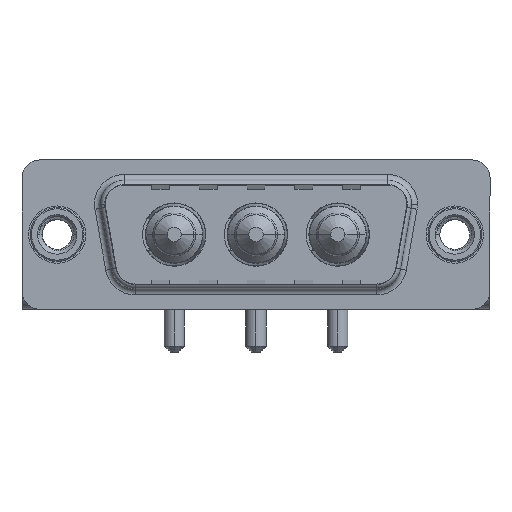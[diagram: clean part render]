
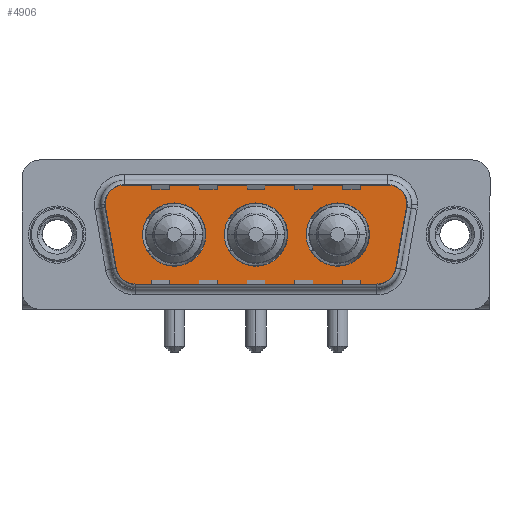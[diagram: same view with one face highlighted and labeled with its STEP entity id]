
A CAD part, top view. The second image highlights one B-rep face of the part: STEP entity #4906.
In plain terms, the highlighted planar face has unit normal (0, 0, 1).
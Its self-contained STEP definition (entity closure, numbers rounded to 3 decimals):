
#16 = DIRECTION ( 'NONE',  ( -1., 0., 0. ) ) ;
#33 = PLANE ( 'NONE',  #1179 ) ;
#123 = DIRECTION ( 'NONE',  ( 0., 0., 1. ) ) ;
#178 = CARTESIAN_POINT ( 'NONE',  ( 6.434, -4.9, 0. ) ) ;
#277 = CIRCLE ( 'NONE', #11703, 2.65 ) ;
#306 = EDGE_CURVE ( 'NONE', #2832, #10535, #11459, .T. ) ;
#308 = EDGE_LOOP ( 'NONE', ( #3486, #2966 ) ) ;
#318 = EDGE_CURVE ( 'NONE', #6557, #2832, #5088, .T. ) ;
#362 = DIRECTION ( 'NONE',  ( -1., 0., 0. ) ) ;
#555 = CARTESIAN_POINT ( 'NONE',  ( 20.85, 0., 0. ) ) ;
#577 = VERTEX_POINT ( 'NONE', #15387 ) ;
#631 = CARTESIAN_POINT ( 'NONE',  ( 5.411, 4.9, 0. ) ) ;
#693 = ORIENTED_EDGE ( 'NONE', *, *, #10812, .F. ) ;
#882 = VERTEX_POINT ( 'NONE', #12918 ) ;
#958 = ORIENTED_EDGE ( 'NONE', *, *, #3874, .T. ) ;
#1175 = ORIENTED_EDGE ( 'NONE', *, *, #6913, .T. ) ;
#1179 = AXIS2_PLACEMENT_3D ( 'NONE', #11768, #9429, #8314 ) ;
#1227 = CARTESIAN_POINT ( 'NONE',  ( 9.8, 0., 0. ) ) ;
#1239 = EDGE_CURVE ( 'NONE', #577, #13368, #1849, .T. ) ;
#1343 = VECTOR ( 'NONE', #4263, 1000. ) ;
#1418 = AXIS2_PLACEMENT_3D ( 'NONE', #13513, #1530, #4067 ) ;
#1456 = DIRECTION ( 'NONE',  ( 1., 0., 0. ) ) ;
#1499 = VERTEX_POINT ( 'NONE', #13284 ) ;
#1530 = DIRECTION ( 'NONE',  ( 0., 0., 1. ) ) ;
#1849 = LINE ( 'NONE', #10267, #1343 ) ;
#1868 = CARTESIAN_POINT ( 'NONE',  ( 16.65, 0., 0. ) ) ;
#1875 = EDGE_CURVE ( 'NONE', #1499, #2037, #9736, .T. ) ;
#2017 = CARTESIAN_POINT ( 'NONE',  ( 27.889, 2.9, 0. ) ) ;
#2037 = VERTEX_POINT ( 'NONE', #4040 ) ;
#2110 = DIRECTION ( 'NONE',  ( 1., 0., 0. ) ) ;
#2243 = DIRECTION ( 'NONE',  ( 0., 0., 1. ) ) ;
#2262 = EDGE_CURVE ( 'NONE', #4130, #882, #277, .T. ) ;
#2265 = EDGE_CURVE ( 'NONE', #13368, #1499, #2493, .T. ) ;
#2266 = FACE_BOUND ( 'NONE', #13736, .T. ) ;
#2382 = CIRCLE ( 'NONE', #14342, 2. ) ;
#2460 = VERTEX_POINT ( 'NONE', #3016 ) ;
#2493 = CIRCLE ( 'NONE', #14206, 2. ) ;
#2589 = ORIENTED_EDGE ( 'NONE', *, *, #1239, .T. ) ;
#2832 = VERTEX_POINT ( 'NONE', #9776 ) ;
#2833 = CARTESIAN_POINT ( 'NONE',  ( 27.889, 2.9, 0. ) ) ;
#2956 = VERTEX_POINT ( 'NONE', #6421 ) ;
#2966 = ORIENTED_EDGE ( 'NONE', *, *, #6146, .F. ) ;
#3016 = CARTESIAN_POINT ( 'NONE',  ( 27.889, 4.9, 0. ) ) ;
#3232 = VECTOR ( 'NONE', #11190, 1000. ) ;
#3486 = ORIENTED_EDGE ( 'NONE', *, *, #13409, .F. ) ;
#3497 = ORIENTED_EDGE ( 'NONE', *, *, #4980, .T. ) ;
#3520 = ORIENTED_EDGE ( 'NONE', *, *, #2262, .F. ) ;
#3670 = CARTESIAN_POINT ( 'NONE',  ( 29.889, 2.9, 0. ) ) ;
#3732 = CARTESIAN_POINT ( 'NONE',  ( 9.8, 0., 0. ) ) ;
#3874 = EDGE_CURVE ( 'NONE', #10535, #2460, #2382, .T. ) ;
#4016 = CARTESIAN_POINT ( 'NONE',  ( 12.45, 0., 0. ) ) ;
#4040 = CARTESIAN_POINT ( 'NONE',  ( 26.866, -4.9, 0. ) ) ;
#4067 = DIRECTION ( 'NONE',  ( 1., 0., 0. ) ) ;
#4130 = VERTEX_POINT ( 'NONE', #7362 ) ;
#4263 = DIRECTION ( 'NONE',  ( 0.174, -0.985, 0. ) ) ;
#4637 = AXIS2_PLACEMENT_3D ( 'NONE', #1227, #10951, #1456 ) ;
#4663 = DIRECTION ( 'NONE',  ( 0., 0., 1. ) ) ;
#4906 = ADVANCED_FACE ( 'NONE', ( #10449, #2266, #8177, #8095 ), #33, .T. ) ;
#4966 = AXIS2_PLACEMENT_3D ( 'NONE', #2833, #8903, #362 ) ;
#4980 = EDGE_CURVE ( 'NONE', #2037, #6557, #6131, .T. ) ;
#5088 = LINE ( 'NONE', #8590, #3232 ) ;
#5361 = VERTEX_POINT ( 'NONE', #631 ) ;
#5397 = CARTESIAN_POINT ( 'NONE',  ( 28.836, -3.247, 0. ) ) ;
#5449 = DIRECTION ( 'NONE',  ( 1., 0., 0. ) ) ;
#5856 = CARTESIAN_POINT ( 'NONE',  ( 5.411, 4.9, 0. ) ) ;
#5874 = CIRCLE ( 'NONE', #1418, 2.65 ) ;
#6131 = CIRCLE ( 'NONE', #14111, 2. ) ;
#6146 = EDGE_CURVE ( 'NONE', #2956, #7357, #10863, .T. ) ;
#6311 = EDGE_CURVE ( 'NONE', #14594, #9166, #5874, .T. ) ;
#6421 = CARTESIAN_POINT ( 'NONE',  ( 7.15, 0., 0. ) ) ;
#6469 = EDGE_LOOP ( 'NONE', ( #3497, #14538, #8035, #958, #12349, #1175, #2589, #9336, #13315 ) ) ;
#6557 = VERTEX_POINT ( 'NONE', #5397 ) ;
#6587 = CIRCLE ( 'NONE', #15316, 2.65 ) ;
#6913 = EDGE_CURVE ( 'NONE', #5361, #577, #10352, .T. ) ;
#7357 = VERTEX_POINT ( 'NONE', #4016 ) ;
#7362 = CARTESIAN_POINT ( 'NONE',  ( 19.3, 0., 0. ) ) ;
#7737 = CARTESIAN_POINT ( 'NONE',  ( 26.15, 0., 0. ) ) ;
#8035 = ORIENTED_EDGE ( 'NONE', *, *, #306, .T. ) ;
#8095 = FACE_OUTER_BOUND ( 'NONE', #6469, .T. ) ;
#8177 = FACE_BOUND ( 'NONE', #308, .T. ) ;
#8199 = DIRECTION ( 'NONE',  ( 1., 0., 0. ) ) ;
#8230 = CARTESIAN_POINT ( 'NONE',  ( 6.434, -2.9, 0. ) ) ;
#8314 = DIRECTION ( 'NONE',  ( 1., 0., 0. ) ) ;
#8431 = LINE ( 'NONE', #5856, #13639 ) ;
#8543 = EDGE_CURVE ( 'NONE', #2460, #5361, #8431, .T. ) ;
#8590 = CARTESIAN_POINT ( 'NONE',  ( 29.859, 2.553, 0. ) ) ;
#8716 = DIRECTION ( 'NONE',  ( 1., 0., 0. ) ) ;
#8863 = CIRCLE ( 'NONE', #11377, 2.65 ) ;
#8903 = DIRECTION ( 'NONE',  ( 0., 0., 1. ) ) ;
#9166 = VERTEX_POINT ( 'NONE', #555 ) ;
#9177 = AXIS2_PLACEMENT_3D ( 'NONE', #11794, #123, #8199 ) ;
#9179 = DIRECTION ( 'NONE',  ( 0., 0., 1. ) ) ;
#9336 = ORIENTED_EDGE ( 'NONE', *, *, #2265, .T. ) ;
#9412 = DIRECTION ( 'NONE',  ( 1., 0., 0. ) ) ;
#9429 = DIRECTION ( 'NONE',  ( 0., 0., 1. ) ) ;
#9504 = CARTESIAN_POINT ( 'NONE',  ( 26.866, -2.9, 0. ) ) ;
#9736 = LINE ( 'NONE', #178, #13416 ) ;
#9776 = CARTESIAN_POINT ( 'NONE',  ( 29.859, 2.553, 0. ) ) ;
#9987 = EDGE_LOOP ( 'NONE', ( #3520, #693 ) ) ;
#10070 = EDGE_CURVE ( 'NONE', #9166, #14594, #10682, .T. ) ;
#10267 = CARTESIAN_POINT ( 'NONE',  ( 3.441, 2.553, 0. ) ) ;
#10352 = CIRCLE ( 'NONE', #13861, 2. ) ;
#10449 = FACE_BOUND ( 'NONE', #9987, .T. ) ;
#10535 = VERTEX_POINT ( 'NONE', #3670 ) ;
#10663 = DIRECTION ( 'NONE',  ( 1., 0., 0. ) ) ;
#10682 = CIRCLE ( 'NONE', #9177, 2.65 ) ;
#10812 = EDGE_CURVE ( 'NONE', #882, #4130, #6587, .T. ) ;
#10863 = CIRCLE ( 'NONE', #4637, 2.65 ) ;
#10951 = DIRECTION ( 'NONE',  ( 0., 0., 1. ) ) ;
#10984 = DIRECTION ( 'NONE',  ( 1., 0., 0. ) ) ;
#11123 = ORIENTED_EDGE ( 'NONE', *, *, #10070, .F. ) ;
#11190 = DIRECTION ( 'NONE',  ( 0.174, 0.985, 0. ) ) ;
#11377 = AXIS2_PLACEMENT_3D ( 'NONE', #3732, #13165, #10984 ) ;
#11459 = CIRCLE ( 'NONE', #4966, 2. ) ;
#11703 = AXIS2_PLACEMENT_3D ( 'NONE', #15348, #4663, #9412 ) ;
#11768 = CARTESIAN_POINT ( 'NONE',  ( 26.866, -2.9, 0. ) ) ;
#11794 = CARTESIAN_POINT ( 'NONE',  ( 23.5, 0., 0. ) ) ;
#11882 = DIRECTION ( 'NONE',  ( -1., 0., 0. ) ) ;
#12349 = ORIENTED_EDGE ( 'NONE', *, *, #8543, .T. ) ;
#12639 = CARTESIAN_POINT ( 'NONE',  ( 5.411, 2.9, 0. ) ) ;
#12709 = DIRECTION ( 'NONE',  ( 0., 0., 1. ) ) ;
#12918 = CARTESIAN_POINT ( 'NONE',  ( 14., 0., 0. ) ) ;
#13010 = DIRECTION ( 'NONE',  ( 0., 0., 1. ) ) ;
#13165 = DIRECTION ( 'NONE',  ( 0., 0., 1. ) ) ;
#13284 = CARTESIAN_POINT ( 'NONE',  ( 6.434, -4.9, 0. ) ) ;
#13315 = ORIENTED_EDGE ( 'NONE', *, *, #1875, .T. ) ;
#13368 = VERTEX_POINT ( 'NONE', #15042 ) ;
#13409 = EDGE_CURVE ( 'NONE', #7357, #2956, #8863, .T. ) ;
#13416 = VECTOR ( 'NONE', #8716, 1000. ) ;
#13429 = ORIENTED_EDGE ( 'NONE', *, *, #6311, .F. ) ;
#13513 = CARTESIAN_POINT ( 'NONE',  ( 23.5, 0., 0. ) ) ;
#13631 = DIRECTION ( 'NONE',  ( 0., 0., 1. ) ) ;
#13639 = VECTOR ( 'NONE', #11882, 1000. ) ;
#13736 = EDGE_LOOP ( 'NONE', ( #13429, #11123 ) ) ;
#13784 = DIRECTION ( 'NONE',  ( -1., 0., 0. ) ) ;
#13861 = AXIS2_PLACEMENT_3D ( 'NONE', #12639, #2243, #10663 ) ;
#14111 = AXIS2_PLACEMENT_3D ( 'NONE', #9504, #13010, #2110 ) ;
#14206 = AXIS2_PLACEMENT_3D ( 'NONE', #8230, #9179, #16 ) ;
#14342 = AXIS2_PLACEMENT_3D ( 'NONE', #2017, #13631, #13784 ) ;
#14538 = ORIENTED_EDGE ( 'NONE', *, *, #318, .T. ) ;
#14594 = VERTEX_POINT ( 'NONE', #7737 ) ;
#15042 = CARTESIAN_POINT ( 'NONE',  ( 4.464, -3.247, 0. ) ) ;
#15316 = AXIS2_PLACEMENT_3D ( 'NONE', #1868, #12709, #5449 ) ;
#15348 = CARTESIAN_POINT ( 'NONE',  ( 16.65, 0., 0. ) ) ;
#15387 = CARTESIAN_POINT ( 'NONE',  ( 3.441, 2.553, 0. ) ) ;
